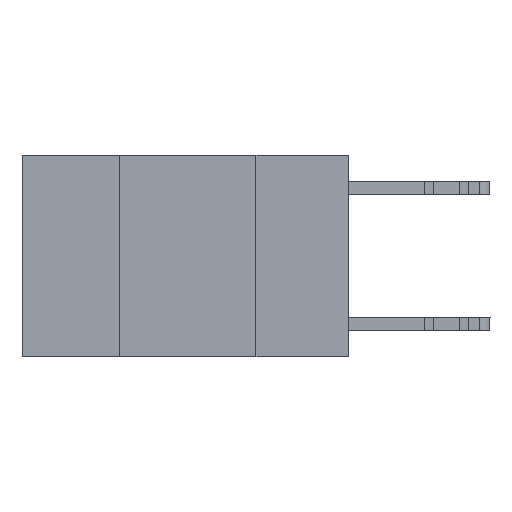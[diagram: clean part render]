
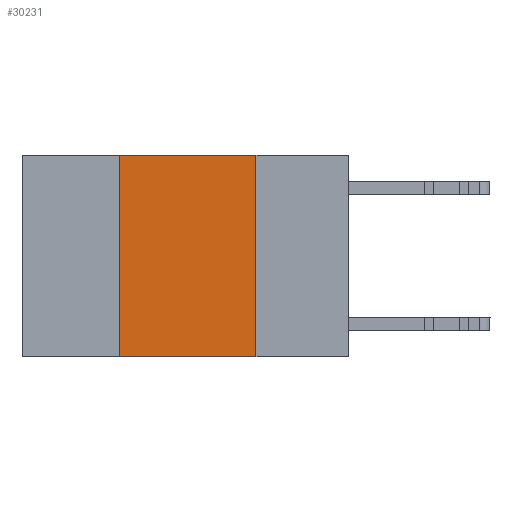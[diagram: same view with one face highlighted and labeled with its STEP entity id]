
A CAD part, left-side view. The second image highlights one B-rep face of the part: STEP entity #30231.
In plain terms, the highlighted planar face has unit normal (-1, 0, 0).
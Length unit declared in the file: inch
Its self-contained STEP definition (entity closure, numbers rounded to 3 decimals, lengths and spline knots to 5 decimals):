
#863 = CARTESIAN_POINT ( 'NONE',  ( 0., 0.42, 0. ) ) ;
#3245 = FACE_OUTER_BOUND ( 'NONE', #30456, .T. ) ;
#4759 = DIRECTION ( 'NONE',  ( 1., 0., 0. ) ) ;
#5505 = VERTEX_POINT ( 'NONE', #21302 ) ;
#6279 = VERTEX_POINT ( 'NONE', #10264 ) ;
#7729 = EDGE_CURVE ( 'NONE', #5505, #6279, #28320, .T. ) ;
#8197 = LINE ( 'NONE', #863, #27309 ) ;
#9195 = CARTESIAN_POINT ( 'NONE',  ( 0., 0.17, 0. ) ) ;
#9943 = LINE ( 'NONE', #9195, #15014 ) ;
#10264 = CARTESIAN_POINT ( 'NONE',  ( 0., 0.17, 0. ) ) ;
#12791 = DIRECTION ( 'NONE',  ( 0., -1., 0. ) ) ;
#14813 = PLANE ( 'NONE',  #28660 ) ;
#15014 = VECTOR ( 'NONE', #31501, 39.37008 ) ;
#15060 = EDGE_CURVE ( 'NONE', #6279, #19167, #9943, .T. ) ;
#15374 = CARTESIAN_POINT ( 'NONE',  ( 0., 0.6, -0.37 ) ) ;
#17890 = DIRECTION ( 'NONE',  ( 0., -1., 0. ) ) ;
#19167 = VERTEX_POINT ( 'NONE', #20073 ) ;
#20073 = CARTESIAN_POINT ( 'NONE',  ( 0., 0.17, -0.37 ) ) ;
#21182 = CARTESIAN_POINT ( 'NONE',  ( 0., 0.42, -0.37 ) ) ;
#21302 = CARTESIAN_POINT ( 'NONE',  ( 0., 0.42, 0. ) ) ;
#22347 = DIRECTION ( 'NONE',  ( 0., 0., -1. ) ) ;
#22370 = EDGE_CURVE ( 'NONE', #31989, #5505, #8197, .T. ) ;
#23403 = VECTOR ( 'NONE', #17890, 39.37008 ) ;
#23436 = EDGE_CURVE ( 'NONE', #31989, #19167, #24190, .T. ) ;
#24190 = LINE ( 'NONE', #15374, #23403 ) ;
#24773 = CARTESIAN_POINT ( 'NONE',  ( 0., 0.6, 0. ) ) ;
#27309 = VECTOR ( 'NONE', #28548, 39.37008 ) ;
#28166 = VECTOR ( 'NONE', #12791, 39.37008 ) ;
#28320 = LINE ( 'NONE', #30125, #28166 ) ;
#28548 = DIRECTION ( 'NONE',  ( 0., 0., 1. ) ) ;
#28660 = AXIS2_PLACEMENT_3D ( 'NONE', #24773, #4759, #22347 ) ;
#29975 = ORIENTED_EDGE ( 'NONE', *, *, #15060, .F. ) ;
#30101 = ORIENTED_EDGE ( 'NONE', *, *, #7729, .F. ) ;
#30125 = CARTESIAN_POINT ( 'NONE',  ( 0., 0.6, 0. ) ) ;
#30231 = ADVANCED_FACE ( 'NONE', ( #3245 ), #14813, .F. ) ;
#30355 = ORIENTED_EDGE ( 'NONE', *, *, #22370, .F. ) ;
#30413 = ORIENTED_EDGE ( 'NONE', *, *, #23436, .T. ) ;
#30456 = EDGE_LOOP ( 'NONE', ( #29975, #30101, #30355, #30413 ) ) ;
#31501 = DIRECTION ( 'NONE',  ( 0., 0., -1. ) ) ;
#31989 = VERTEX_POINT ( 'NONE', #21182 ) ;
